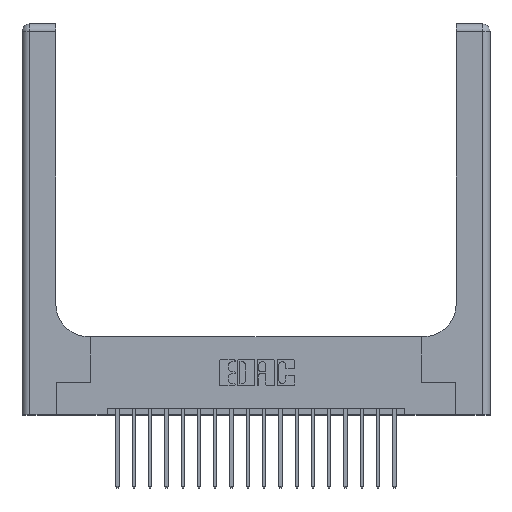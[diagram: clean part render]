
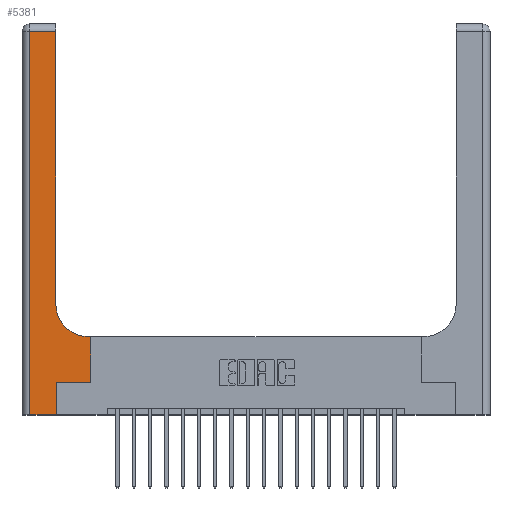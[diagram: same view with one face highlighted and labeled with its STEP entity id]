
A CAD part, top view. The second image highlights one B-rep face of the part: STEP entity #5381.
In plain terms, the highlighted planar face has unit normal (0, 0, 1).
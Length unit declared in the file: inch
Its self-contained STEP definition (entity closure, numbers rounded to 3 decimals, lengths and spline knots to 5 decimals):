
#982 = DIRECTION ( 'NONE',  ( 0., 0., -1. ) ) ;
#1639 = CARTESIAN_POINT ( 'NONE',  ( 0.26, 0.6, 0.37 ) ) ;
#2114 = ORIENTED_EDGE ( 'NONE', *, *, #16563, .T. ) ;
#2537 = EDGE_CURVE ( 'NONE', #7676, #10839, #20078, .T. ) ;
#2715 = VECTOR ( 'NONE', #13812, 39.37008 ) ;
#2753 = CARTESIAN_POINT ( 'NONE',  ( 0.51, 0.85, 0.37 ) ) ;
#2806 = CARTESIAN_POINT ( 'NONE',  ( 0., 2.94, 0.37 ) ) ;
#3017 = VECTOR ( 'NONE', #14065, 39.37008 ) ;
#3500 = VERTEX_POINT ( 'NONE', #13076 ) ;
#4428 = CARTESIAN_POINT ( 'NONE',  ( 0.528, 0.25, 0.37 ) ) ;
#4909 = FACE_OUTER_BOUND ( 'NONE', #12410, .T. ) ;
#5031 = VERTEX_POINT ( 'NONE', #8640 ) ;
#5381 = ADVANCED_FACE ( 'NONE', ( #4909 ), #7500, .F. ) ;
#5421 = EDGE_CURVE ( 'NONE', #10839, #11664, #6847, .T. ) ;
#5567 = EDGE_CURVE ( 'NONE', #9608, #16938, #15819, .T. ) ;
#5718 = DIRECTION ( 'NONE',  ( -1., 0., 0. ) ) ;
#6094 = DIRECTION ( 'NONE',  ( 0., 1., 0. ) ) ;
#6207 = ORIENTED_EDGE ( 'NONE', *, *, #2537, .T. ) ;
#6566 = CARTESIAN_POINT ( 'NONE',  ( 0.265, 0.25, 0.37 ) ) ;
#6675 = VECTOR ( 'NONE', #9278, 39.37008 ) ;
#6829 = VECTOR ( 'NONE', #9847, 39.37008 ) ;
#6847 = LINE ( 'NONE', #15371, #2715 ) ;
#7054 = ORIENTED_EDGE ( 'NONE', *, *, #17568, .T. ) ;
#7500 = PLANE ( 'NONE',  #19914 ) ;
#7676 = VERTEX_POINT ( 'NONE', #8066 ) ;
#7826 = ORIENTED_EDGE ( 'NONE', *, *, #14348, .T. ) ;
#8066 = CARTESIAN_POINT ( 'NONE',  ( 0.06, 2.94, 0.37 ) ) ;
#8346 = EDGE_CURVE ( 'NONE', #8493, #5031, #13528, .T. ) ;
#8393 = CARTESIAN_POINT ( 'NONE',  ( 0.265, 0., 0.37 ) ) ;
#8493 = VERTEX_POINT ( 'NONE', #14038 ) ;
#8579 = VECTOR ( 'NONE', #5718, 39.37008 ) ;
#8640 = CARTESIAN_POINT ( 'NONE',  ( 0.26, 2.94, 0.37 ) ) ;
#8680 = ORIENTED_EDGE ( 'NONE', *, *, #5567, .T. ) ;
#8907 = CIRCLE ( 'NONE', #17664, 0.25 ) ;
#9094 = VERTEX_POINT ( 'NONE', #16830 ) ;
#9096 = CARTESIAN_POINT ( 'NONE',  ( 0., 3., 0.37 ) ) ;
#9113 = VECTOR ( 'NONE', #6094, 39.37008 ) ;
#9215 = VECTOR ( 'NONE', #17015, 39.37008 ) ;
#9278 = DIRECTION ( 'NONE',  ( 1., 0., 0. ) ) ;
#9608 = VERTEX_POINT ( 'NONE', #4428 ) ;
#9847 = DIRECTION ( 'NONE',  ( 0., 1., 0. ) ) ;
#9917 = CARTESIAN_POINT ( 'NONE',  ( 0.528, 0.25, 0.37 ) ) ;
#10839 = VERTEX_POINT ( 'NONE', #17386 ) ;
#11270 = EDGE_CURVE ( 'NONE', #5031, #7676, #20054, .T. ) ;
#11660 = LINE ( 'NONE', #1639, #9215 ) ;
#11664 = VERTEX_POINT ( 'NONE', #8393 ) ;
#12172 = ORIENTED_EDGE ( 'NONE', *, *, #8346, .T. ) ;
#12410 = EDGE_LOOP ( 'NONE', ( #12172, #19054, #6207, #13734, #2114, #7054, #8680, #7826, #12716 ) ) ;
#12716 = ORIENTED_EDGE ( 'NONE', *, *, #15597, .T. ) ;
#13076 = CARTESIAN_POINT ( 'NONE',  ( 0.265, 0.25, 0.37 ) ) ;
#13528 = LINE ( 'NONE', #13849, #9113 ) ;
#13734 = ORIENTED_EDGE ( 'NONE', *, *, #5421, .T. ) ;
#13812 = DIRECTION ( 'NONE',  ( 1., 0., 0. ) ) ;
#13849 = CARTESIAN_POINT ( 'NONE',  ( 0.26, 3., 0.37 ) ) ;
#13945 = DIRECTION ( 'NONE',  ( 0., 0., -1. ) ) ;
#14038 = CARTESIAN_POINT ( 'NONE',  ( 0.26, 0.85, 0.37 ) ) ;
#14065 = DIRECTION ( 'NONE',  ( 0., -1., 0. ) ) ;
#14348 = EDGE_CURVE ( 'NONE', #16938, #9094, #11660, .T. ) ;
#14975 = VECTOR ( 'NONE', #17767, 39.37008 ) ;
#15180 = DIRECTION ( 'NONE',  ( 1., 0., 0. ) ) ;
#15371 = CARTESIAN_POINT ( 'NONE',  ( 0., 0., 0.37 ) ) ;
#15488 = CARTESIAN_POINT ( 'NONE',  ( 0.528, 0.6, 0.37 ) ) ;
#15515 = DIRECTION ( 'NONE',  ( -1., 0., 0. ) ) ;
#15597 = EDGE_CURVE ( 'NONE', #9094, #8493, #8907, .T. ) ;
#15819 = LINE ( 'NONE', #9917, #6829 ) ;
#15923 = LINE ( 'NONE', #6566, #6675 ) ;
#16133 = CARTESIAN_POINT ( 'NONE',  ( 0.265, 0., 0.37 ) ) ;
#16563 = EDGE_CURVE ( 'NONE', #11664, #3500, #16681, .T. ) ;
#16681 = LINE ( 'NONE', #16133, #14975 ) ;
#16830 = CARTESIAN_POINT ( 'NONE',  ( 0.51, 0.6, 0.37 ) ) ;
#16930 = CARTESIAN_POINT ( 'NONE',  ( 0.06, 3., 0.37 ) ) ;
#16938 = VERTEX_POINT ( 'NONE', #15488 ) ;
#17015 = DIRECTION ( 'NONE',  ( -1., 0., 0. ) ) ;
#17386 = CARTESIAN_POINT ( 'NONE',  ( 0.06, 0., 0.37 ) ) ;
#17568 = EDGE_CURVE ( 'NONE', #3500, #9608, #15923, .T. ) ;
#17664 = AXIS2_PLACEMENT_3D ( 'NONE', #2753, #982, #15180 ) ;
#17767 = DIRECTION ( 'NONE',  ( 0., 1., 0. ) ) ;
#19054 = ORIENTED_EDGE ( 'NONE', *, *, #11270, .T. ) ;
#19914 = AXIS2_PLACEMENT_3D ( 'NONE', #9096, #13945, #15515 ) ;
#20054 = LINE ( 'NONE', #2806, #8579 ) ;
#20078 = LINE ( 'NONE', #16930, #3017 ) ;
